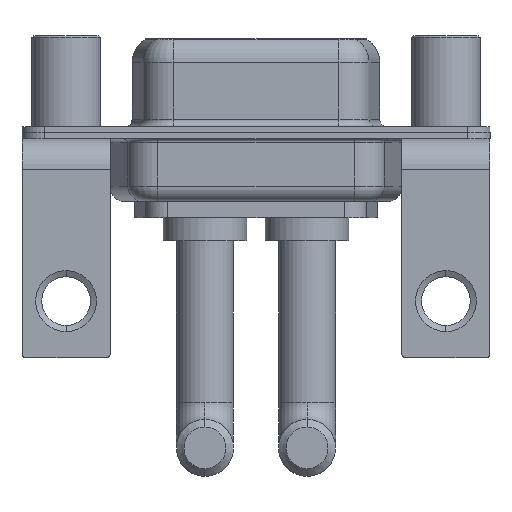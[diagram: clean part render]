
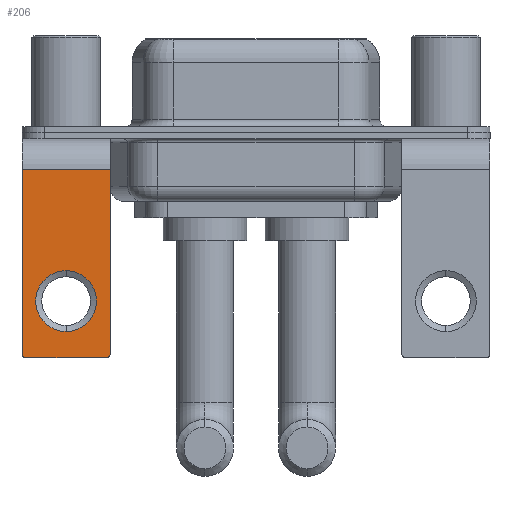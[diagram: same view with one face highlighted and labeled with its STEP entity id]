
A CAD part, front view. The second image highlights one B-rep face of the part: STEP entity #206.
In plain terms, the highlighted planar face has unit normal (0, -1, 0).
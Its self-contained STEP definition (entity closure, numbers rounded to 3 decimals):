
#16 = EDGE_LOOP ( 'NONE', ( #4809, #1907, #5403, #8912, #14656, #10068 ) ) ;
#206 = ADVANCED_FACE ( 'NONE', ( #7395, #566 ), #9626, .F. ) ;
#324 = DIRECTION ( 'NONE',  ( 0., 0., -1. ) ) ;
#566 = FACE_OUTER_BOUND ( 'NONE', #16, .T. ) ;
#712 = VERTEX_POINT ( 'NONE', #6259 ) ;
#795 = VERTEX_POINT ( 'NONE', #4865 ) ;
#883 = CIRCLE ( 'NONE', #4910, 2. ) ;
#1178 = EDGE_CURVE ( 'NONE', #2302, #712, #14573, .T. ) ;
#1251 = VERTEX_POINT ( 'NONE', #8933 ) ;
#1318 = DIRECTION ( 'NONE',  ( 0., -1., 0. ) ) ;
#1450 = CARTESIAN_POINT ( 'NONE',  ( 2.65, -6.25, -14.8 ) ) ;
#1907 = ORIENTED_EDGE ( 'NONE', *, *, #12603, .T. ) ;
#2302 = VERTEX_POINT ( 'NONE', #1450 ) ;
#2534 = CARTESIAN_POINT ( 'NONE',  ( 0., -6.25, -11.07 ) ) ;
#2607 = DIRECTION ( 'NONE',  ( 0., 1., 0. ) ) ;
#2654 = EDGE_CURVE ( 'NONE', #795, #11362, #13684, .T. ) ;
#2774 = VECTOR ( 'NONE', #8040, 1000. ) ;
#2878 = CARTESIAN_POINT ( 'NONE',  ( 2.9, -6.25, -2.4 ) ) ;
#3202 = AXIS2_PLACEMENT_3D ( 'NONE', #6737, #11327, #5697 ) ;
#3523 = CARTESIAN_POINT ( 'NONE',  ( 2.9, -6.25, -2.4 ) ) ;
#3581 = DIRECTION ( 'NONE',  ( 0., 0., 1. ) ) ;
#3722 = CARTESIAN_POINT ( 'NONE',  ( -2.9, -6.25, -14.55 ) ) ;
#4809 = ORIENTED_EDGE ( 'NONE', *, *, #6632, .T. ) ;
#4865 = CARTESIAN_POINT ( 'NONE',  ( 2.9, -6.25, -2.4 ) ) ;
#4910 = AXIS2_PLACEMENT_3D ( 'NONE', #12787, #2607, #3581 ) ;
#4951 = CIRCLE ( 'NONE', #10165, 2. ) ;
#5383 = ORIENTED_EDGE ( 'NONE', *, *, #10471, .T. ) ;
#5403 = ORIENTED_EDGE ( 'NONE', *, *, #1178, .F. ) ;
#5697 = DIRECTION ( 'NONE',  ( 0., 0., 1. ) ) ;
#5743 = ORIENTED_EDGE ( 'NONE', *, *, #9084, .T. ) ;
#6186 = CARTESIAN_POINT ( 'NONE',  ( -2.9, -6.25, -2.4 ) ) ;
#6259 = CARTESIAN_POINT ( 'NONE',  ( -2.65, -6.25, -14.8 ) ) ;
#6428 = CIRCLE ( 'NONE', #12588, 0.25 ) ;
#6632 = EDGE_CURVE ( 'NONE', #8918, #9152, #10564, .T. ) ;
#6737 = CARTESIAN_POINT ( 'NONE',  ( 2.65, -6.25, -14.55 ) ) ;
#6884 = VECTOR ( 'NONE', #9587, 1000. ) ;
#6986 = DIRECTION ( 'NONE',  ( 0., 1., 0. ) ) ;
#7101 = EDGE_CURVE ( 'NONE', #2302, #11362, #9593, .T. ) ;
#7156 = CARTESIAN_POINT ( 'NONE',  ( -2.9, -6.25, -2.4 ) ) ;
#7395 = FACE_BOUND ( 'NONE', #12404, .T. ) ;
#7426 = CARTESIAN_POINT ( 'NONE',  ( 2.9, -6.25, -2.4 ) ) ;
#7772 = VECTOR ( 'NONE', #10380, 1000. ) ;
#8040 = DIRECTION ( 'NONE',  ( 0., 0., -1. ) ) ;
#8091 = CARTESIAN_POINT ( 'NONE',  ( 2.9, -6.25, -14.8 ) ) ;
#8912 = ORIENTED_EDGE ( 'NONE', *, *, #7101, .T. ) ;
#8918 = VERTEX_POINT ( 'NONE', #6186 ) ;
#8933 = CARTESIAN_POINT ( 'NONE',  ( 0., -6.25, -9.07 ) ) ;
#9084 = EDGE_CURVE ( 'NONE', #10202, #1251, #883, .T. ) ;
#9152 = VERTEX_POINT ( 'NONE', #3722 ) ;
#9204 = CARTESIAN_POINT ( 'NONE',  ( -2.65, -6.25, -14.55 ) ) ;
#9587 = DIRECTION ( 'NONE',  ( -1., 0., 0. ) ) ;
#9593 = CIRCLE ( 'NONE', #3202, 0.25 ) ;
#9626 = PLANE ( 'NONE',  #11768 ) ;
#10068 = ORIENTED_EDGE ( 'NONE', *, *, #12111, .T. ) ;
#10165 = AXIS2_PLACEMENT_3D ( 'NONE', #2534, #6986, #11587 ) ;
#10202 = VERTEX_POINT ( 'NONE', #12051 ) ;
#10380 = DIRECTION ( 'NONE',  ( -1., 0., 0. ) ) ;
#10471 = EDGE_CURVE ( 'NONE', #1251, #10202, #4951, .T. ) ;
#10564 = LINE ( 'NONE', #7156, #11204 ) ;
#11204 = VECTOR ( 'NONE', #324, 1000. ) ;
#11327 = DIRECTION ( 'NONE',  ( 0., -1., 0. ) ) ;
#11362 = VERTEX_POINT ( 'NONE', #14667 ) ;
#11587 = DIRECTION ( 'NONE',  ( 0., 0., 1. ) ) ;
#11768 = AXIS2_PLACEMENT_3D ( 'NONE', #2878, #14151, #11926 ) ;
#11926 = DIRECTION ( 'NONE',  ( 0., 0., 1. ) ) ;
#12051 = CARTESIAN_POINT ( 'NONE',  ( 0., -6.25, -13.07 ) ) ;
#12111 = EDGE_CURVE ( 'NONE', #795, #8918, #14265, .T. ) ;
#12404 = EDGE_LOOP ( 'NONE', ( #5743, #5383 ) ) ;
#12588 = AXIS2_PLACEMENT_3D ( 'NONE', #9204, #1318, #13591 ) ;
#12603 = EDGE_CURVE ( 'NONE', #9152, #712, #6428, .T. ) ;
#12787 = CARTESIAN_POINT ( 'NONE',  ( 0., -6.25, -11.07 ) ) ;
#13591 = DIRECTION ( 'NONE',  ( 0., 0., 1. ) ) ;
#13684 = LINE ( 'NONE', #3523, #2774 ) ;
#14151 = DIRECTION ( 'NONE',  ( 0., 1., 0. ) ) ;
#14265 = LINE ( 'NONE', #7426, #6884 ) ;
#14573 = LINE ( 'NONE', #8091, #7772 ) ;
#14656 = ORIENTED_EDGE ( 'NONE', *, *, #2654, .F. ) ;
#14667 = CARTESIAN_POINT ( 'NONE',  ( 2.9, -6.25, -14.55 ) ) ;
